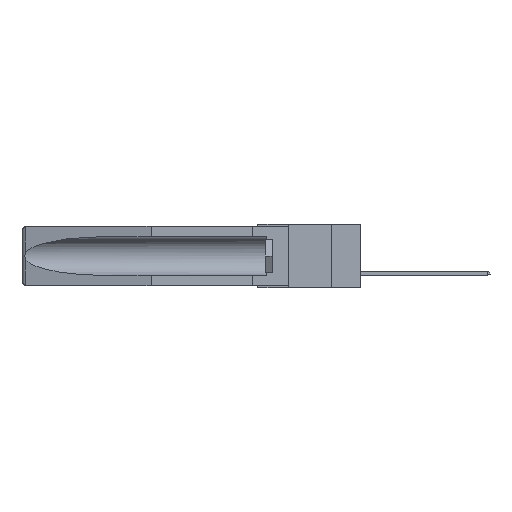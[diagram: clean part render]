
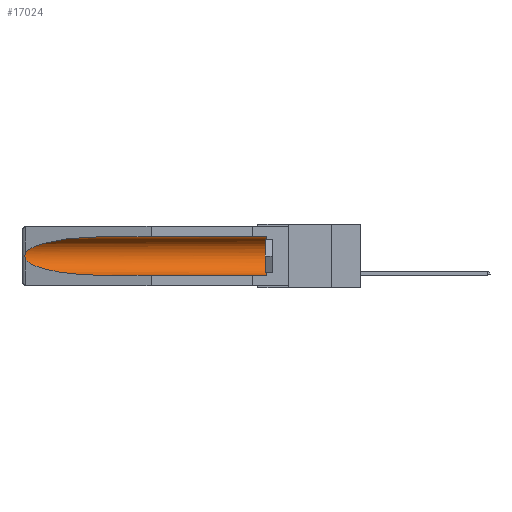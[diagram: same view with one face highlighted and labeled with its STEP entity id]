
A CAD part, left-side view. The second image highlights one B-rep face of the part: STEP entity #17024.
In plain terms, the highlighted cylindrical face has radius 2.857 mm (diameter 5.715 mm), a partial arc.
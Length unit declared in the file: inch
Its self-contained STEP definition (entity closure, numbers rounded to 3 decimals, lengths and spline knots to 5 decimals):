
#136 = B_SPLINE_CURVE_WITH_KNOTS ( 'NONE', 3,
 ( #23277, #19745, #10802, #1444, #14066, #16560, #5442, #11043, #10898, #3883 ),
 .UNSPECIFIED., .F., .F.,
 ( 4, 2, 2, 2, 4 ),
 ( 0., 0.00029, 0.00058, 0.00087, 0.00117 ),
 .UNSPECIFIED. ) ;
#766 = EDGE_CURVE ( 'NONE', #23327, #6141, #20814, .T. ) ;
#1248 = CARTESIAN_POINT ( 'NONE',  ( 0.155, -0.30754, -0.1715 ) ) ;
#1444 = CARTESIAN_POINT ( 'NONE',  ( 0.2673, 1.5327, -0.16383 ) ) ;
#1681 = AXIS2_PLACEMENT_3D ( 'NONE', #3735, #5476, #18186 ) ;
#1872 =( BOUNDED_CURVE ( )  B_SPLINE_CURVE ( 3, ( #19486, #23173, #17587, #8607 ),
 .UNSPECIFIED., .F., .F. ) 
 B_SPLINE_CURVE_WITH_KNOTS ( ( 4, 4 ),
 ( 4.71239, 6.08839 ),
 .UNSPECIFIED. ) 
 CURVE ( )  GEOMETRIC_REPRESENTATION_ITEM ( )  RATIONAL_B_SPLINE_CURVE ( ( 1., 0.848, 0.848, 1. ) ) 
 REPRESENTATION_ITEM ( '' )  );
#2177 = EDGE_CURVE ( 'NONE', #20541, #13550, #1872, .T. ) ;
#2259 = DIRECTION ( 'NONE',  ( 0., 1., 0. ) ) ;
#2537 = CARTESIAN_POINT ( 'NONE',  ( 0.155, 0.126, -0.284 ) ) ;
#3735 = CARTESIAN_POINT ( 'NONE',  ( 0.155, 0.126, -0.1715 ) ) ;
#3883 = CARTESIAN_POINT ( 'NONE',  ( 0.26537, 1.52718, -0.19328 ) ) ;
#3935 = ORIENTED_EDGE ( 'NONE', *, *, #19469, .T. ) ;
#4339 = ORIENTED_EDGE ( 'NONE', *, *, #11181, .T. ) ;
#4370 = AXIS2_PLACEMENT_3D ( 'NONE', #1248, #10768, #10322 ) ;
#5442 = CARTESIAN_POINT ( 'NONE',  ( 0.2673, 1.53269, -0.17917 ) ) ;
#5476 = DIRECTION ( 'NONE',  ( 0., -1., 0. ) ) ;
#5535 = CARTESIAN_POINT ( 'NONE',  ( 0.25451, 1.48313, -0.24835 ) ) ;
#5669 = VERTEX_POINT ( 'NONE', #16361 ) ;
#6141 = VERTEX_POINT ( 'NONE', #14252 ) ;
#6325 = CARTESIAN_POINT ( 'NONE',  ( 0.26537, 1.52718, -0.19328 ) ) ;
#6632 = VECTOR ( 'NONE', #2259, 39.37008 ) ;
#6676 = CARTESIAN_POINT ( 'NONE',  ( 0.155, -0.30754, -0.284 ) ) ;
#8268 = CYLINDRICAL_SURFACE ( 'NONE', #4370, 0.1125 ) ;
#8607 = CARTESIAN_POINT ( 'NONE',  ( 0.26537, 1.52718, -0.14972 ) ) ;
#10322 = DIRECTION ( 'NONE',  ( 0., 0., 1. ) ) ;
#10768 = DIRECTION ( 'NONE',  ( 0., 1., 0. ) ) ;
#10802 = CARTESIAN_POINT ( 'NONE',  ( 0.26654, 1.53092, -0.15636 ) ) ;
#10898 = CARTESIAN_POINT ( 'NONE',  ( 0.26597, 1.5296, -0.19026 ) ) ;
#11010 = CIRCLE ( 'NONE', #1681, 0.1125 ) ;
#11043 = CARTESIAN_POINT ( 'NONE',  ( 0.26655, 1.53094, -0.18657 ) ) ;
#11181 = EDGE_CURVE ( 'NONE', #23327, #5669, #11010, .T. ) ;
#12692 = CARTESIAN_POINT ( 'NONE',  ( 0.26537, 1.52718, -0.19328 ) ) ;
#12911 = CARTESIAN_POINT ( 'NONE',  ( 0.155, 1.07973, -0.059 ) ) ;
#13308 = EDGE_CURVE ( 'NONE', #14154, #6141, #21848, .T. ) ;
#13550 = VERTEX_POINT ( 'NONE', #20894 ) ;
#13904 = DIRECTION ( 'NONE',  ( 0., 1., 0. ) ) ;
#14066 = CARTESIAN_POINT ( 'NONE',  ( 0.2675, 1.53308, -0.16763 ) ) ;
#14154 = VERTEX_POINT ( 'NONE', #6325 ) ;
#14252 = CARTESIAN_POINT ( 'NONE',  ( 0.155, 1.07973, -0.284 ) ) ;
#14286 = EDGE_LOOP ( 'NONE', ( #22488, #3935, #14791, #19924, #4339, #17230 ) ) ;
#14791 = ORIENTED_EDGE ( 'NONE', *, *, #13308, .T. ) ;
#15314 = FACE_OUTER_BOUND ( 'NONE', #14286, .T. ) ;
#16223 = EDGE_CURVE ( 'NONE', #5669, #20541, #19310, .T. ) ;
#16361 = CARTESIAN_POINT ( 'NONE',  ( 0.155, 0.126, -0.059 ) ) ;
#16560 = CARTESIAN_POINT ( 'NONE',  ( 0.2675, 1.53308, -0.17534 ) ) ;
#17024 = ADVANCED_FACE ( 'NONE', ( #15314 ), #8268, .F. ) ;
#17230 = ORIENTED_EDGE ( 'NONE', *, *, #16223, .T. ) ;
#17587 = CARTESIAN_POINT ( 'NONE',  ( 0.25451, 1.48313, -0.09465 ) ) ;
#18186 = DIRECTION ( 'NONE',  ( 0., 0., 1. ) ) ;
#18445 = CARTESIAN_POINT ( 'NONE',  ( 0.155, -0.30754, -0.059 ) ) ;
#18519 = VECTOR ( 'NONE', #13904, 39.37008 ) ;
#19310 = LINE ( 'NONE', #18445, #6632 ) ;
#19469 = EDGE_CURVE ( 'NONE', #13550, #14154, #136, .T. ) ;
#19486 = CARTESIAN_POINT ( 'NONE',  ( 0.155, 1.07973, -0.059 ) ) ;
#19745 = CARTESIAN_POINT ( 'NONE',  ( 0.26597, 1.52961, -0.15275 ) ) ;
#19924 = ORIENTED_EDGE ( 'NONE', *, *, #766, .F. ) ;
#19993 = CARTESIAN_POINT ( 'NONE',  ( 0.155, 1.07973, -0.284 ) ) ;
#20145 = CARTESIAN_POINT ( 'NONE',  ( 0.21114, 1.30732, -0.284 ) ) ;
#20541 = VERTEX_POINT ( 'NONE', #12911 ) ;
#20814 = LINE ( 'NONE', #6676, #18519 ) ;
#20894 = CARTESIAN_POINT ( 'NONE',  ( 0.26537, 1.52718, -0.14972 ) ) ;
#21848 =( BOUNDED_CURVE ( )  B_SPLINE_CURVE ( 3, ( #12692, #5535, #20145, #19993 ),
 .UNSPECIFIED., .F., .F. ) 
 B_SPLINE_CURVE_WITH_KNOTS ( ( 4, 4 ),
 ( 0.1948, 1.5708 ),
 .UNSPECIFIED. ) 
 CURVE ( )  GEOMETRIC_REPRESENTATION_ITEM ( )  RATIONAL_B_SPLINE_CURVE ( ( 1., 0.848, 0.848, 1. ) ) 
 REPRESENTATION_ITEM ( '' )  );
#22488 = ORIENTED_EDGE ( 'NONE', *, *, #2177, .T. ) ;
#23173 = CARTESIAN_POINT ( 'NONE',  ( 0.21114, 1.30732, -0.059 ) ) ;
#23277 = CARTESIAN_POINT ( 'NONE',  ( 0.26537, 1.52718, -0.14972 ) ) ;
#23327 = VERTEX_POINT ( 'NONE', #2537 ) ;
